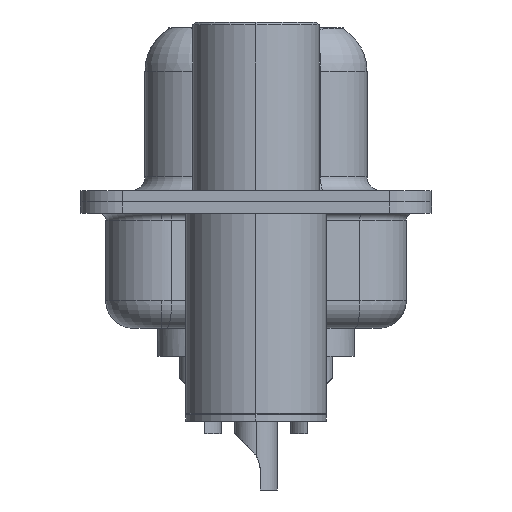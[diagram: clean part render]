
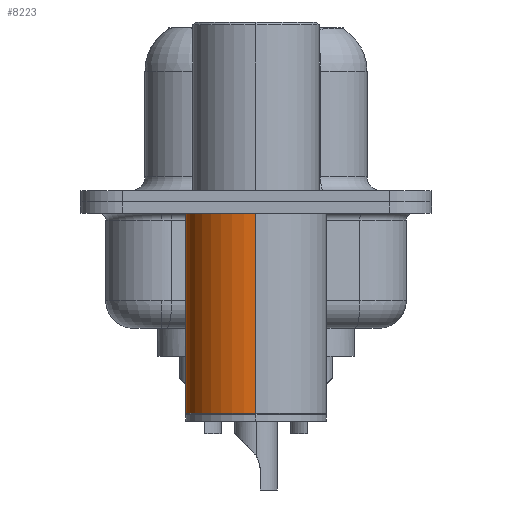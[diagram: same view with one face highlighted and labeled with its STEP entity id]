
A CAD part, left-side view. The second image highlights one B-rep face of the part: STEP entity #8223.
In plain terms, the highlighted cylindrical face has radius 2.5 mm (diameter 5 mm), a partial arc.
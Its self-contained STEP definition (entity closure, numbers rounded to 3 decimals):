
#719 = DIRECTION ( 'NONE',  ( 0., 0., 1. ) ) ;
#3647 = ORIENTED_EDGE ( 'NONE', *, *, #12514, .F. ) ;
#4757 = EDGE_LOOP ( 'NONE', ( #17775, #19568, #19524, #3647 ) ) ;
#5017 = AXIS2_PLACEMENT_3D ( 'NONE', #11256, #24138, #11751 ) ;
#5258 = LINE ( 'NONE', #13314, #21079 ) ;
#5693 = LINE ( 'NONE', #8338, #8887 ) ;
#5709 = DIRECTION ( 'NONE',  ( 0., 0., 1. ) ) ;
#6222 = VERTEX_POINT ( 'NONE', #10363 ) ;
#7010 = CARTESIAN_POINT ( 'NONE',  ( 2.5, 0., -0.4 ) ) ;
#7790 = CARTESIAN_POINT ( 'NONE',  ( -2.5, 0., -7.525 ) ) ;
#8223 = ADVANCED_FACE ( 'NONE', ( #21327 ), #26477, .T. ) ;
#8338 = CARTESIAN_POINT ( 'NONE',  ( 2.5, 0., 0.581 ) ) ;
#8887 = VECTOR ( 'NONE', #31193, 1000. ) ;
#9130 = VERTEX_POINT ( 'NONE', #7010 ) ;
#10363 = CARTESIAN_POINT ( 'NONE',  ( 2.5, 0., -7.525 ) ) ;
#11256 = CARTESIAN_POINT ( 'NONE',  ( 0., 0., 0.581 ) ) ;
#11751 = DIRECTION ( 'NONE',  ( 1., 0., 0. ) ) ;
#12287 = CIRCLE ( 'NONE', #30810, 2.5 ) ;
#12514 = EDGE_CURVE ( 'NONE', #6222, #9130, #5693, .T. ) ;
#13314 = CARTESIAN_POINT ( 'NONE',  ( -2.5, 0., 0.581 ) ) ;
#16373 = EDGE_CURVE ( 'NONE', #9130, #27674, #12287, .T. ) ;
#17624 = CARTESIAN_POINT ( 'NONE',  ( 0., 0., -7.525 ) ) ;
#17775 = ORIENTED_EDGE ( 'NONE', *, *, #32339, .T. ) ;
#18051 = AXIS2_PLACEMENT_3D ( 'NONE', #17624, #5709, #20913 ) ;
#19524 = ORIENTED_EDGE ( 'NONE', *, *, #16373, .F. ) ;
#19546 = CARTESIAN_POINT ( 'NONE',  ( -2.5, 0., -0.4 ) ) ;
#19568 = ORIENTED_EDGE ( 'NONE', *, *, #30543, .T. ) ;
#20913 = DIRECTION ( 'NONE',  ( 1., 0., 0. ) ) ;
#21079 = VECTOR ( 'NONE', #719, 1000. ) ;
#21327 = FACE_OUTER_BOUND ( 'NONE', #4757, .T. ) ;
#21418 = VERTEX_POINT ( 'NONE', #7790 ) ;
#21735 = CIRCLE ( 'NONE', #18051, 2.5 ) ;
#22569 = DIRECTION ( 'NONE',  ( 0., 0., 1. ) ) ;
#24138 = DIRECTION ( 'NONE',  ( 0., 0., 1. ) ) ;
#26477 = CYLINDRICAL_SURFACE ( 'NONE', #5017, 2.5 ) ;
#27674 = VERTEX_POINT ( 'NONE', #19546 ) ;
#28374 = CARTESIAN_POINT ( 'NONE',  ( 0., 0., -0.4 ) ) ;
#30539 = DIRECTION ( 'NONE',  ( 1., 0., 0. ) ) ;
#30543 = EDGE_CURVE ( 'NONE', #21418, #27674, #5258, .T. ) ;
#30810 = AXIS2_PLACEMENT_3D ( 'NONE', #28374, #22569, #30539 ) ;
#31193 = DIRECTION ( 'NONE',  ( 0., 0., 1. ) ) ;
#32339 = EDGE_CURVE ( 'NONE', #6222, #21418, #21735, .T. ) ;
